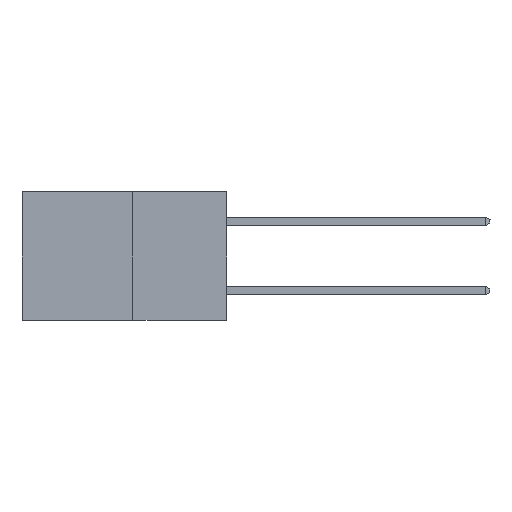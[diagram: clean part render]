
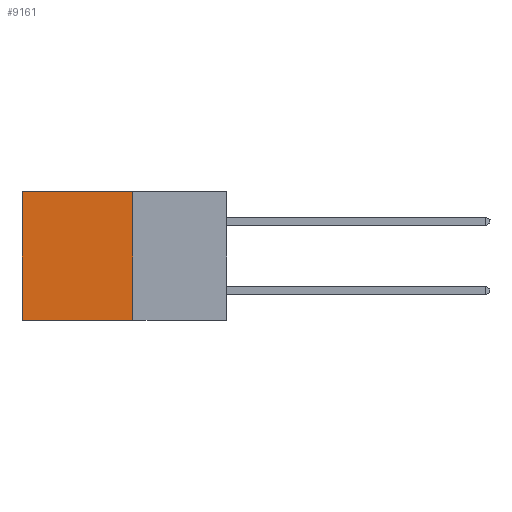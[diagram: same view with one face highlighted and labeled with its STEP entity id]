
A CAD part, left-side view. The second image highlights one B-rep face of the part: STEP entity #9161.
In plain terms, the highlighted planar face has unit normal (-1, 0, 0).
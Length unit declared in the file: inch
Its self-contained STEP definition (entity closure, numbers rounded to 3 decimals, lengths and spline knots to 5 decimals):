
#754 = VERTEX_POINT ( 'NONE', #15576 ) ;
#1834 = EDGE_CURVE ( 'NONE', #18170, #23760, #21575, .T. ) ;
#4217 = CARTESIAN_POINT ( 'NONE',  ( 0.277, 0.27, -0.37 ) ) ;
#4329 = CARTESIAN_POINT ( 'NONE',  ( 0.277, 0.59, 0. ) ) ;
#4790 = LINE ( 'NONE', #18223, #14588 ) ;
#6615 = LINE ( 'NONE', #4217, #11201 ) ;
#6776 = ORIENTED_EDGE ( 'NONE', *, *, #8307, .T. ) ;
#7264 = CARTESIAN_POINT ( 'NONE',  ( 0.277, 0.27, -0.37 ) ) ;
#8307 = EDGE_CURVE ( 'NONE', #23760, #754, #4790, .T. ) ;
#8913 = DIRECTION ( 'NONE',  ( 0., 1., 0. ) ) ;
#9156 = ORIENTED_EDGE ( 'NONE', *, *, #18574, .F. ) ;
#9161 = ADVANCED_FACE ( 'NONE', ( #10592 ), #20289, .F. ) ;
#10592 = FACE_OUTER_BOUND ( 'NONE', #18741, .T. ) ;
#11096 = DIRECTION ( 'NONE',  ( 0., 0., -1. ) ) ;
#11201 = VECTOR ( 'NONE', #19744, 39.37008 ) ;
#14588 = VECTOR ( 'NONE', #18391, 39.37008 ) ;
#15289 = ORIENTED_EDGE ( 'NONE', *, *, #21535, .F. ) ;
#15323 = CARTESIAN_POINT ( 'NONE',  ( 0.277, 0.27, 0. ) ) ;
#15576 = CARTESIAN_POINT ( 'NONE',  ( 0.277, 0.59, -0.37 ) ) ;
#16515 = VECTOR ( 'NONE', #8913, 39.37008 ) ;
#16700 = LINE ( 'NONE', #7264, #17300 ) ;
#17217 = VERTEX_POINT ( 'NONE', #20020 ) ;
#17300 = VECTOR ( 'NONE', #11096, 39.37008 ) ;
#18170 = VERTEX_POINT ( 'NONE', #19527 ) ;
#18223 = CARTESIAN_POINT ( 'NONE',  ( 0.277, 0.59, -0.37 ) ) ;
#18391 = DIRECTION ( 'NONE',  ( 0., 0., -1. ) ) ;
#18397 = ORIENTED_EDGE ( 'NONE', *, *, #1834, .T. ) ;
#18574 = EDGE_CURVE ( 'NONE', #18170, #17217, #16700, .T. ) ;
#18741 = EDGE_LOOP ( 'NONE', ( #6776, #15289, #9156, #18397 ) ) ;
#19527 = CARTESIAN_POINT ( 'NONE',  ( 0.277, 0.27, 0. ) ) ;
#19528 = AXIS2_PLACEMENT_3D ( 'NONE', #20402, #20089, #20037 ) ;
#19744 = DIRECTION ( 'NONE',  ( 0., 1., 0. ) ) ;
#20020 = CARTESIAN_POINT ( 'NONE',  ( 0.277, 0.27, -0.37 ) ) ;
#20037 = DIRECTION ( 'NONE',  ( 0., 0., -1. ) ) ;
#20089 = DIRECTION ( 'NONE',  ( 1., 0., 0. ) ) ;
#20289 = PLANE ( 'NONE',  #19528 ) ;
#20402 = CARTESIAN_POINT ( 'NONE',  ( 0.277, 0.27, -0.37 ) ) ;
#21535 = EDGE_CURVE ( 'NONE', #17217, #754, #6615, .T. ) ;
#21575 = LINE ( 'NONE', #15323, #16515 ) ;
#23760 = VERTEX_POINT ( 'NONE', #4329 ) ;
